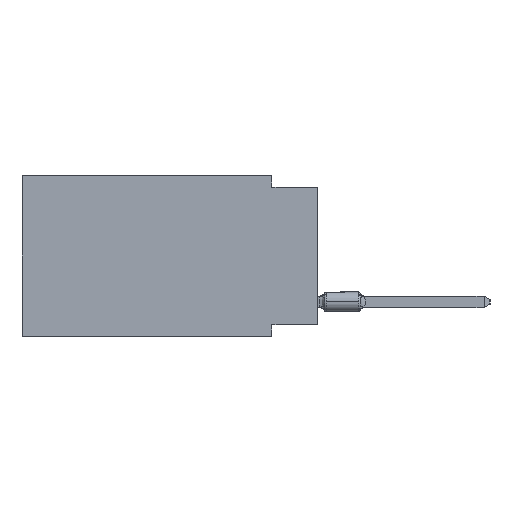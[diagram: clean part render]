
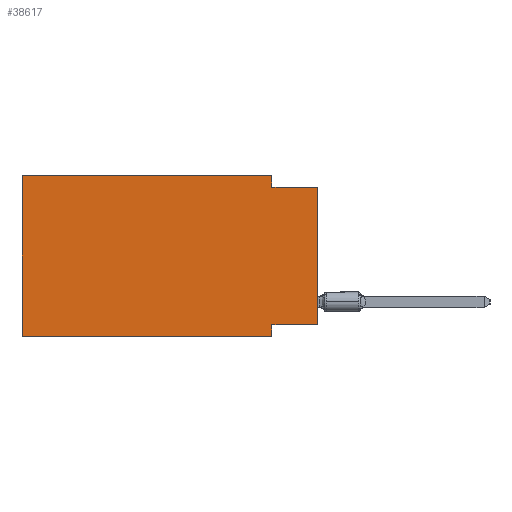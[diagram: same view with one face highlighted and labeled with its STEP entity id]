
A CAD part, left-side view. The second image highlights one B-rep face of the part: STEP entity #38617.
In plain terms, the highlighted planar face has unit normal (-1, 0, 0).
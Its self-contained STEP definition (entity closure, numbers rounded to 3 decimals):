
#842 = CARTESIAN_POINT ( 'NONE',  ( 0., 2.54, -0.635 ) ) ;
#1790 = ORIENTED_EDGE ( 'NONE', *, *, #5482, .F. ) ;
#1840 = DIRECTION ( 'NONE',  ( 0., 0., 1. ) ) ;
#1926 = ORIENTED_EDGE ( 'NONE', *, *, #24474, .F. ) ;
#2196 = EDGE_CURVE ( 'NONE', #2805, #57753, #25826, .T. ) ;
#2728 = DIRECTION ( 'NONE',  ( 0., 0., -1. ) ) ;
#2805 = VERTEX_POINT ( 'NONE', #52599 ) ;
#3259 = LINE ( 'NONE', #25685, #18424 ) ;
#3694 = VECTOR ( 'NONE', #34961, 1000. ) ;
#3869 = VECTOR ( 'NONE', #5163, 1000. ) ;
#4020 = CARTESIAN_POINT ( 'NONE',  ( 0., 0., -8.255 ) ) ;
#4650 = CARTESIAN_POINT ( 'NONE',  ( 0., 2.54, 0. ) ) ;
#5163 = DIRECTION ( 'NONE',  ( 0., 0., -1. ) ) ;
#5482 = EDGE_CURVE ( 'NONE', #16850, #49829, #37011, .T. ) ;
#5923 = LINE ( 'NONE', #24204, #24208 ) ;
#6312 = ORIENTED_EDGE ( 'NONE', *, *, #20234, .T. ) ;
#6600 = CARTESIAN_POINT ( 'NONE',  ( 0., 0., -8.255 ) ) ;
#8113 = VECTOR ( 'NONE', #54656, 1000. ) ;
#11506 = EDGE_CURVE ( 'NONE', #57753, #15032, #3259, .T. ) ;
#12981 = EDGE_CURVE ( 'NONE', #25199, #2805, #28401, .T. ) ;
#14290 = ORIENTED_EDGE ( 'NONE', *, *, #12981, .F. ) ;
#15032 = VERTEX_POINT ( 'NONE', #842 ) ;
#16241 = DIRECTION ( 'NONE',  ( 0., 0., 1. ) ) ;
#16737 = VERTEX_POINT ( 'NONE', #6600 ) ;
#16850 = VERTEX_POINT ( 'NONE', #45228 ) ;
#17366 = CARTESIAN_POINT ( 'NONE',  ( 0., 16.383, -8.89 ) ) ;
#17803 = ORIENTED_EDGE ( 'NONE', *, *, #11506, .F. ) ;
#18424 = VECTOR ( 'NONE', #52228, 1000. ) ;
#18639 = VECTOR ( 'NONE', #1840, 1000. ) ;
#19402 = DIRECTION ( 'NONE',  ( 0., -1., 0. ) ) ;
#20234 = EDGE_CURVE ( 'NONE', #25199, #49829, #32132, .T. ) ;
#20691 = CARTESIAN_POINT ( 'NONE',  ( 0., 2.54, -8.89 ) ) ;
#21394 = CARTESIAN_POINT ( 'NONE',  ( 0., 16.383, 0. ) ) ;
#24116 = EDGE_LOOP ( 'NONE', ( #53804, #1926, #17803, #47613, #14290, #6312, #1790, #36371 ) ) ;
#24204 = CARTESIAN_POINT ( 'NONE',  ( 0., 0., 0. ) ) ;
#24208 = VECTOR ( 'NONE', #16241, 1000. ) ;
#24474 = EDGE_CURVE ( 'NONE', #15032, #58275, #45518, .T. ) ;
#24848 = VECTOR ( 'NONE', #19402, 1000. ) ;
#25149 = FACE_OUTER_BOUND ( 'NONE', #24116, .T. ) ;
#25199 = VERTEX_POINT ( 'NONE', #17366 ) ;
#25452 = DIRECTION ( 'NONE',  ( 1., 0., 0. ) ) ;
#25685 = CARTESIAN_POINT ( 'NONE',  ( 0., 2.54, 0. ) ) ;
#25826 = LINE ( 'NONE', #21394, #3694 ) ;
#28401 = LINE ( 'NONE', #29282, #18639 ) ;
#29282 = CARTESIAN_POINT ( 'NONE',  ( 0., 16.383, 0. ) ) ;
#30460 = EDGE_CURVE ( 'NONE', #16737, #16850, #40289, .T. ) ;
#31160 = DIRECTION ( 'NONE',  ( 0., 1., 0. ) ) ;
#32132 = LINE ( 'NONE', #40689, #24848 ) ;
#32304 = CARTESIAN_POINT ( 'NONE',  ( 0., 2.54, -8.89 ) ) ;
#33398 = VECTOR ( 'NONE', #31160, 1000. ) ;
#34879 = PLANE ( 'NONE',  #39601 ) ;
#34961 = DIRECTION ( 'NONE',  ( 0., -1., 0. ) ) ;
#36371 = ORIENTED_EDGE ( 'NONE', *, *, #30460, .F. ) ;
#37011 = LINE ( 'NONE', #32304, #3869 ) ;
#38617 = ADVANCED_FACE ( 'NONE', ( #25149 ), #34879, .F. ) ;
#39601 = AXIS2_PLACEMENT_3D ( 'NONE', #52872, #25452, #2728 ) ;
#40289 = LINE ( 'NONE', #4020, #33398 ) ;
#40689 = CARTESIAN_POINT ( 'NONE',  ( 0., 16.383, -8.89 ) ) ;
#41385 = CARTESIAN_POINT ( 'NONE',  ( 0., 0., -0.635 ) ) ;
#45228 = CARTESIAN_POINT ( 'NONE',  ( 0., 2.54, -8.255 ) ) ;
#45518 = LINE ( 'NONE', #41385, #8113 ) ;
#45570 = CARTESIAN_POINT ( 'NONE',  ( 0., 0., -0.635 ) ) ;
#47613 = ORIENTED_EDGE ( 'NONE', *, *, #2196, .F. ) ;
#48782 = EDGE_CURVE ( 'NONE', #16737, #58275, #5923, .T. ) ;
#49829 = VERTEX_POINT ( 'NONE', #20691 ) ;
#52228 = DIRECTION ( 'NONE',  ( 0., 0., -1. ) ) ;
#52599 = CARTESIAN_POINT ( 'NONE',  ( 0., 16.383, 0. ) ) ;
#52872 = CARTESIAN_POINT ( 'NONE',  ( 0., 16.383, 0. ) ) ;
#53804 = ORIENTED_EDGE ( 'NONE', *, *, #48782, .T. ) ;
#54656 = DIRECTION ( 'NONE',  ( 0., -1., 0. ) ) ;
#57753 = VERTEX_POINT ( 'NONE', #4650 ) ;
#58275 = VERTEX_POINT ( 'NONE', #45570 ) ;
